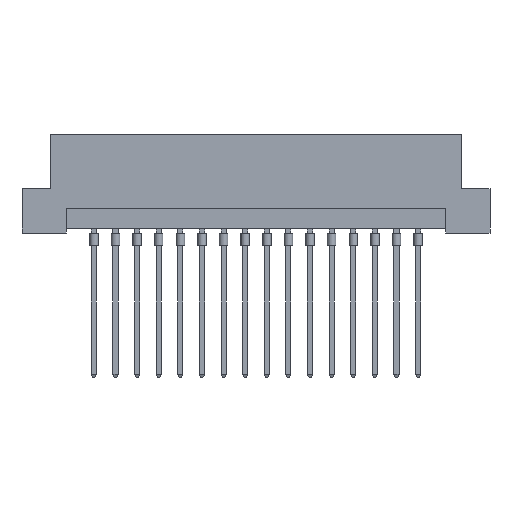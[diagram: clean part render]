
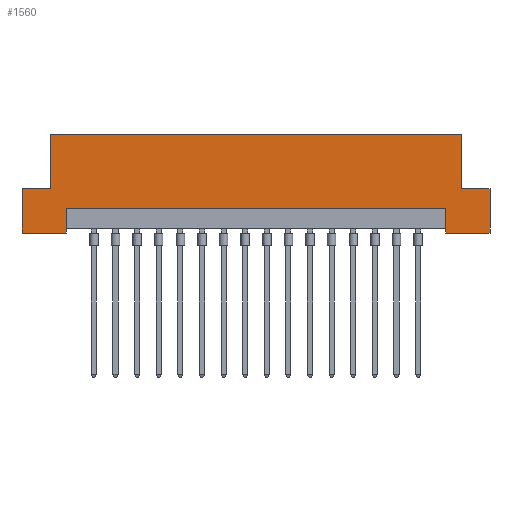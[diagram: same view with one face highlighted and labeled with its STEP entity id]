
A CAD part, front view. The second image highlights one B-rep face of the part: STEP entity #1560.
In plain terms, the highlighted planar face has unit normal (0, -1, 0).
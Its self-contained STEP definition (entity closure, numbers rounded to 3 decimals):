
#91 = CARTESIAN_POINT ( 'NONE',  ( -22.3, 0., 2.9 ) ) ;
#301 = DIRECTION ( 'NONE',  ( 1., 0., 0. ) ) ;
#575 = CARTESIAN_POINT ( 'NONE',  ( 27.5, 0., 5.2 ) ) ;
#822 = DIRECTION ( 'NONE',  ( 0., 1., 0. ) ) ;
#995 = EDGE_CURVE ( 'NONE', #4718, #3178, #3921, .T. ) ;
#1298 = LINE ( 'NONE', #575, #8538 ) ;
#1416 = ORIENTED_EDGE ( 'NONE', *, *, #4181, .F. ) ;
#1560 = ADVANCED_FACE ( 'NONE', ( #6663 ), #2849, .F. ) ;
#1660 = CARTESIAN_POINT ( 'NONE',  ( 27.5, 0., 0. ) ) ;
#1759 = LINE ( 'NONE', #7025, #6404 ) ;
#1889 = EDGE_CURVE ( 'NONE', #7443, #4158, #8872, .T. ) ;
#1969 = ORIENTED_EDGE ( 'NONE', *, *, #8571, .F. ) ;
#1981 = VERTEX_POINT ( 'NONE', #6068 ) ;
#2127 = EDGE_CURVE ( 'NONE', #7537, #4946, #1759, .T. ) ;
#2134 = VECTOR ( 'NONE', #8309, 1000. ) ;
#2327 = CARTESIAN_POINT ( 'NONE',  ( -24.2, 0., 5.2 ) ) ;
#2366 = CARTESIAN_POINT ( 'NONE',  ( -27.5, 0., 5.2 ) ) ;
#2523 = CARTESIAN_POINT ( 'NONE',  ( -27.5, 0., 5.2 ) ) ;
#2849 = PLANE ( 'NONE',  #8715 ) ;
#2973 = VERTEX_POINT ( 'NONE', #6902 ) ;
#2987 = CARTESIAN_POINT ( 'NONE',  ( -27.5, 0., 11.6 ) ) ;
#3082 = CARTESIAN_POINT ( 'NONE',  ( -27.5, 0., 0. ) ) ;
#3178 = VERTEX_POINT ( 'NONE', #3418 ) ;
#3185 = EDGE_CURVE ( 'NONE', #7043, #2973, #8595, .T. ) ;
#3347 = DIRECTION ( 'NONE',  ( 0., 0., -1. ) ) ;
#3418 = CARTESIAN_POINT ( 'NONE',  ( 22.3, 0., 0. ) ) ;
#3470 = ORIENTED_EDGE ( 'NONE', *, *, #4522, .F. ) ;
#3484 = ORIENTED_EDGE ( 'NONE', *, *, #7192, .F. ) ;
#3537 = CARTESIAN_POINT ( 'NONE',  ( 22.3, 0., 0.5 ) ) ;
#3564 = ORIENTED_EDGE ( 'NONE', *, *, #7156, .F. ) ;
#3569 = CARTESIAN_POINT ( 'NONE',  ( 27.5, 0., 5.2 ) ) ;
#3620 = ORIENTED_EDGE ( 'NONE', *, *, #3884, .F. ) ;
#3795 = VERTEX_POINT ( 'NONE', #2327 ) ;
#3851 = VERTEX_POINT ( 'NONE', #2523 ) ;
#3884 = EDGE_CURVE ( 'NONE', #1981, #2973, #7596, .T. ) ;
#3921 = LINE ( 'NONE', #3537, #5026 ) ;
#4010 = VECTOR ( 'NONE', #8990, 1000. ) ;
#4098 = ORIENTED_EDGE ( 'NONE', *, *, #995, .T. ) ;
#4158 = VERTEX_POINT ( 'NONE', #6760 ) ;
#4181 = EDGE_CURVE ( 'NONE', #4158, #3178, #6046, .T. ) ;
#4270 = DIRECTION ( 'NONE',  ( -1., 0., 0. ) ) ;
#4407 = VECTOR ( 'NONE', #4612, 1000. ) ;
#4423 = VECTOR ( 'NONE', #6748, 1000. ) ;
#4447 = LINE ( 'NONE', #7351, #7993 ) ;
#4522 = EDGE_CURVE ( 'NONE', #7043, #7443, #1298, .T. ) ;
#4612 = DIRECTION ( 'NONE',  ( 0., 0., -1. ) ) ;
#4701 = CARTESIAN_POINT ( 'NONE',  ( -27.5, 0., 11.6 ) ) ;
#4718 = VERTEX_POINT ( 'NONE', #8732 ) ;
#4946 = VERTEX_POINT ( 'NONE', #8188 ) ;
#5009 = LINE ( 'NONE', #6451, #5418 ) ;
#5026 = VECTOR ( 'NONE', #7121, 1000. ) ;
#5199 = EDGE_CURVE ( 'NONE', #4946, #8895, #5009, .T. ) ;
#5418 = VECTOR ( 'NONE', #4270, 1000. ) ;
#5732 = VECTOR ( 'NONE', #301, 1000. ) ;
#5874 = ORIENTED_EDGE ( 'NONE', *, *, #3185, .T. ) ;
#5916 = VECTOR ( 'NONE', #7191, 1000. ) ;
#6046 = LINE ( 'NONE', #3082, #4010 ) ;
#6068 = CARTESIAN_POINT ( 'NONE',  ( -24.2, 0., 11.6 ) ) ;
#6079 = EDGE_LOOP ( 'NONE', ( #1969, #4098, #1416, #8766, #3470, #5874, #3620, #3564, #3484, #8018, #8465, #9309 ) ) ;
#6143 = LINE ( 'NONE', #2366, #2134 ) ;
#6310 = VECTOR ( 'NONE', #6962, 1000. ) ;
#6404 = VECTOR ( 'NONE', #3347, 1000. ) ;
#6451 = CARTESIAN_POINT ( 'NONE',  ( -27.5, 0., 0. ) ) ;
#6471 = DIRECTION ( 'NONE',  ( 1., 0., 0. ) ) ;
#6663 = FACE_OUTER_BOUND ( 'NONE', #6079, .T. ) ;
#6748 = DIRECTION ( 'NONE',  ( -1., 0., 0. ) ) ;
#6760 = CARTESIAN_POINT ( 'NONE',  ( 27.5, 0., 0. ) ) ;
#6902 = CARTESIAN_POINT ( 'NONE',  ( 24.2, 0., 11.6 ) ) ;
#6962 = DIRECTION ( 'NONE',  ( 0., 0., 1. ) ) ;
#7025 = CARTESIAN_POINT ( 'NONE',  ( -22.3, 0., 0.5 ) ) ;
#7043 = VERTEX_POINT ( 'NONE', #8075 ) ;
#7108 = EDGE_CURVE ( 'NONE', #8895, #3851, #4447, .T. ) ;
#7121 = DIRECTION ( 'NONE',  ( 0., 0., -1. ) ) ;
#7156 = EDGE_CURVE ( 'NONE', #3795, #1981, #8121, .T. ) ;
#7191 = DIRECTION ( 'NONE',  ( 0., 0., 1. ) ) ;
#7192 = EDGE_CURVE ( 'NONE', #3851, #3795, #6143, .T. ) ;
#7351 = CARTESIAN_POINT ( 'NONE',  ( -27.5, 0., 0. ) ) ;
#7443 = VERTEX_POINT ( 'NONE', #3569 ) ;
#7448 = DIRECTION ( 'NONE',  ( 0., 0., 1. ) ) ;
#7537 = VERTEX_POINT ( 'NONE', #91 ) ;
#7590 = CARTESIAN_POINT ( 'NONE',  ( -24.2, 0., 5.2 ) ) ;
#7596 = LINE ( 'NONE', #4701, #5732 ) ;
#7868 = CARTESIAN_POINT ( 'NONE',  ( 24.2, 0., 5.2 ) ) ;
#7993 = VECTOR ( 'NONE', #7448, 1000. ) ;
#8018 = ORIENTED_EDGE ( 'NONE', *, *, #7108, .F. ) ;
#8075 = CARTESIAN_POINT ( 'NONE',  ( 24.2, 0., 5.2 ) ) ;
#8121 = LINE ( 'NONE', #7590, #6310 ) ;
#8188 = CARTESIAN_POINT ( 'NONE',  ( -22.3, 0., 0. ) ) ;
#8200 = CARTESIAN_POINT ( 'NONE',  ( 22.3, 0., 2.9 ) ) ;
#8309 = DIRECTION ( 'NONE',  ( 1., 0., 0. ) ) ;
#8465 = ORIENTED_EDGE ( 'NONE', *, *, #5199, .F. ) ;
#8538 = VECTOR ( 'NONE', #6471, 1000. ) ;
#8571 = EDGE_CURVE ( 'NONE', #4718, #7537, #8982, .T. ) ;
#8595 = LINE ( 'NONE', #7868, #5916 ) ;
#8715 = AXIS2_PLACEMENT_3D ( 'NONE', #2987, #822, #9468 ) ;
#8732 = CARTESIAN_POINT ( 'NONE',  ( 22.3, 0., 2.9 ) ) ;
#8766 = ORIENTED_EDGE ( 'NONE', *, *, #1889, .F. ) ;
#8872 = LINE ( 'NONE', #1660, #4407 ) ;
#8895 = VERTEX_POINT ( 'NONE', #9272 ) ;
#8982 = LINE ( 'NONE', #8200, #4423 ) ;
#8990 = DIRECTION ( 'NONE',  ( -1., 0., 0. ) ) ;
#9272 = CARTESIAN_POINT ( 'NONE',  ( -27.5, 0., 0. ) ) ;
#9309 = ORIENTED_EDGE ( 'NONE', *, *, #2127, .F. ) ;
#9468 = DIRECTION ( 'NONE',  ( 0., 0., 1. ) ) ;
